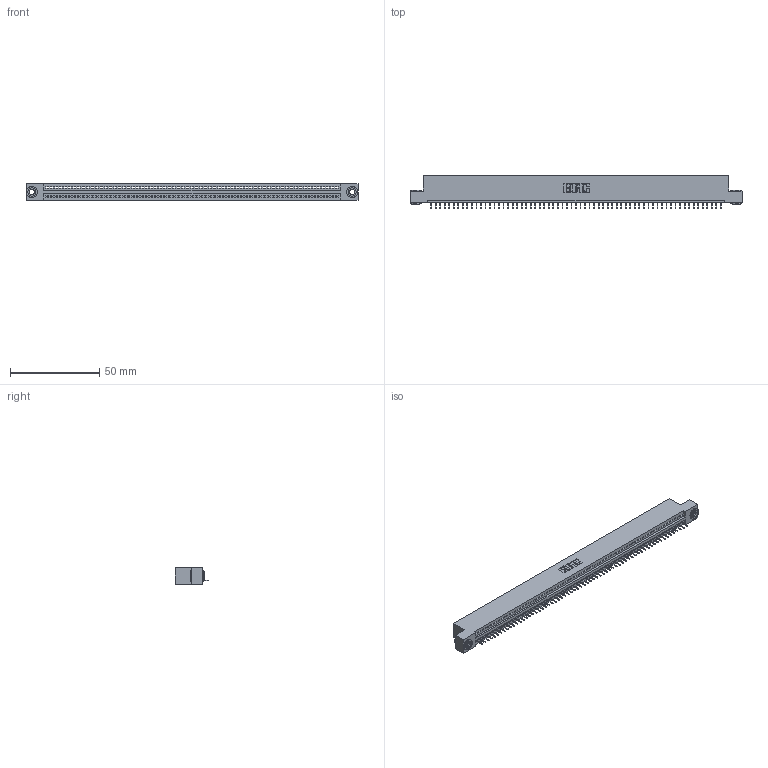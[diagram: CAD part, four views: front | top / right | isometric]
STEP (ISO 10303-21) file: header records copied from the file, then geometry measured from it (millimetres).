
FILE_DESCRIPTION (( 'STEP AP203' ), '1' );
FILE_NAME ('845-065-525-103.STEP', '2020-09-23T18:21:23', ( '' ), ( '' ), 'SwSTEP 2.0', 'SolidWorks 2020', '' );
FILE_SCHEMA (( 'CONFIG_CONTROL_DESIGN' ));
Length unit declared in the file: inch
Products named in the file (4): 845 Part_Flush Mounting Lugs - 0.156 Dia-TH; 845-065-525-103; 345-250-002_345-250-002-102; 345-292-001_345-293-125
Assembly tree (68 placements, depth 2):
  845-065-525-103
    845 Part_Flush Mounting Lugs - 0.156 Dia-TH
    345-292-001_345-293-125  x65
    345-250-002_345-250-002-102  x2
Bounding box: 186.31 x 18.72 x 9.4 mm (x, y, z)
Volume: 17638.2 mm3; surface area: 23081.7 mm2
Topology: 68 solids, 68 shells, 4194 faces, 12117 edges, 7814 vertices
Faces by surface type: plane 3080, cylinder 1106, cone 8
Entity records: 46548 total; most frequent: CARTESIAN_POINT 8038, ORIENTED_EDGE 8030, DIRECTION 7019, EDGE_CURVE 4015, LINE 3603, VECTOR 3603, VERTEX_POINT 2670, AXIS2_PLACEMENT_3D 1708
